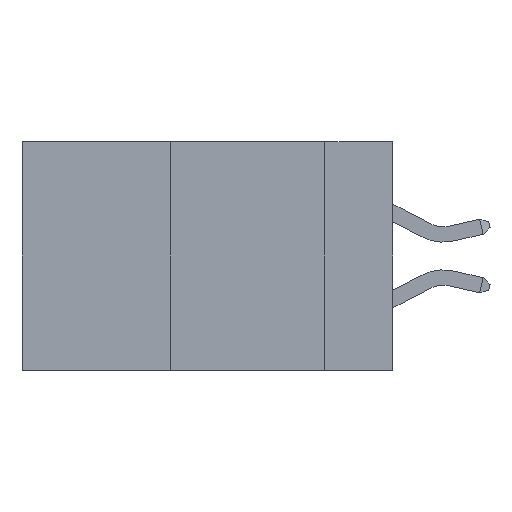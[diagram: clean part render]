
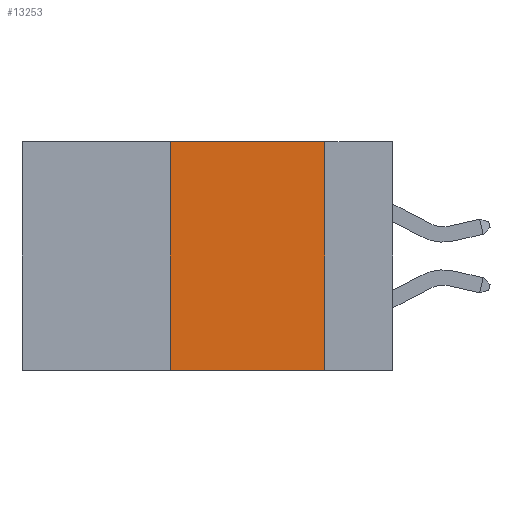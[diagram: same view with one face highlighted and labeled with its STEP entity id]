
A CAD part, left-side view. The second image highlights one B-rep face of the part: STEP entity #13253.
In plain terms, the highlighted planar face has unit normal (-1, 0, 0).
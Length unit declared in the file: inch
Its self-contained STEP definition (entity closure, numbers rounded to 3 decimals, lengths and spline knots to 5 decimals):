
#316 = EDGE_LOOP ( 'NONE', ( #15569, #6443, #4542, #6889 ) ) ;
#433 = EDGE_CURVE ( 'NONE', #9041, #12085, #976, .T. ) ;
#976 = LINE ( 'NONE', #16382, #11995 ) ;
#1111 = VERTEX_POINT ( 'NONE', #11747 ) ;
#1195 = PLANE ( 'NONE',  #5033 ) ;
#1271 = DIRECTION ( 'NONE',  ( 0., -1., 0. ) ) ;
#2534 = VECTOR ( 'NONE', #13305, 39.37008 ) ;
#2656 = DIRECTION ( 'NONE',  ( 1., 0., 0. ) ) ;
#3834 = VECTOR ( 'NONE', #12251, 39.37008 ) ;
#4542 = ORIENTED_EDGE ( 'NONE', *, *, #7217, .F. ) ;
#4619 = CARTESIAN_POINT ( 'NONE',  ( 0., 0.36, -0.37 ) ) ;
#5033 = AXIS2_PLACEMENT_3D ( 'NONE', #9771, #2656, #12670 ) ;
#5222 = FACE_OUTER_BOUND ( 'NONE', #316, .T. ) ;
#6387 = EDGE_CURVE ( 'NONE', #1111, #16919, #13922, .T. ) ;
#6405 = VECTOR ( 'NONE', #12305, 39.37008 ) ;
#6443 = ORIENTED_EDGE ( 'NONE', *, *, #6387, .F. ) ;
#6889 = ORIENTED_EDGE ( 'NONE', *, *, #433, .T. ) ;
#7136 = LINE ( 'NONE', #10797, #3834 ) ;
#7217 = EDGE_CURVE ( 'NONE', #9041, #1111, #7136, .T. ) ;
#9041 = VERTEX_POINT ( 'NONE', #4619 ) ;
#9771 = CARTESIAN_POINT ( 'NONE',  ( 0., 0.6, 0. ) ) ;
#10259 = LINE ( 'NONE', #17807, #6405 ) ;
#10797 = CARTESIAN_POINT ( 'NONE',  ( 0., 0.36, 0. ) ) ;
#11131 = EDGE_CURVE ( 'NONE', #16919, #12085, #10259, .T. ) ;
#11747 = CARTESIAN_POINT ( 'NONE',  ( 0., 0.36, 0. ) ) ;
#11898 = CARTESIAN_POINT ( 'NONE',  ( 0., 0.6, 0. ) ) ;
#11995 = VECTOR ( 'NONE', #1271, 39.37008 ) ;
#12085 = VERTEX_POINT ( 'NONE', #17233 ) ;
#12251 = DIRECTION ( 'NONE',  ( 0., 0., 1. ) ) ;
#12305 = DIRECTION ( 'NONE',  ( 0., 0., -1. ) ) ;
#12670 = DIRECTION ( 'NONE',  ( 0., 0., -1. ) ) ;
#13253 = ADVANCED_FACE ( 'NONE', ( #5222 ), #1195, .F. ) ;
#13305 = DIRECTION ( 'NONE',  ( 0., -1., 0. ) ) ;
#13920 = CARTESIAN_POINT ( 'NONE',  ( 0., 0.11, 0. ) ) ;
#13922 = LINE ( 'NONE', #11898, #2534 ) ;
#15569 = ORIENTED_EDGE ( 'NONE', *, *, #11131, .F. ) ;
#16382 = CARTESIAN_POINT ( 'NONE',  ( 0., 0.6, -0.37 ) ) ;
#16919 = VERTEX_POINT ( 'NONE', #13920 ) ;
#17233 = CARTESIAN_POINT ( 'NONE',  ( 0., 0.11, -0.37 ) ) ;
#17807 = CARTESIAN_POINT ( 'NONE',  ( 0., 0.11, 0. ) ) ;
